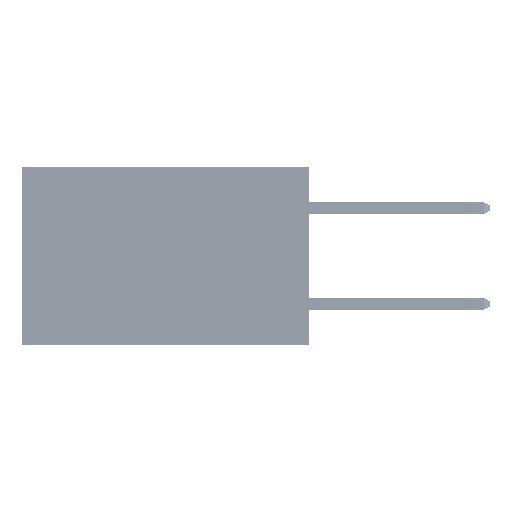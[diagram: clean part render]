
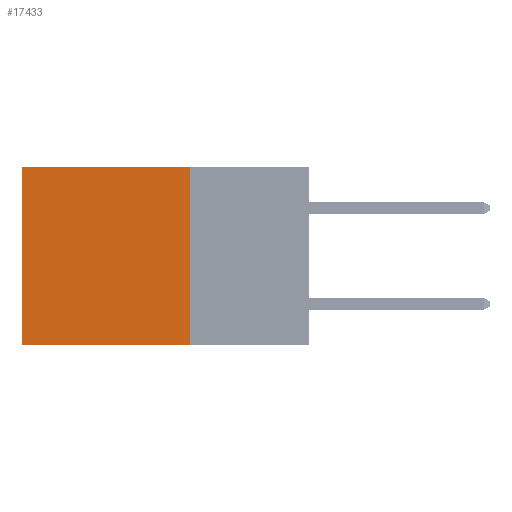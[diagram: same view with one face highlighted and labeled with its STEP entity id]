
A CAD part, left-side view. The second image highlights one B-rep face of the part: STEP entity #17433.
In plain terms, the highlighted planar face has unit normal (-1, 0, 0).
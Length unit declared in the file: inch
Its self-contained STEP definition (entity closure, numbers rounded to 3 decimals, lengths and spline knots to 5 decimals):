
#2884 = CARTESIAN_POINT ( 'NONE',  ( 0.2875, 0.25, -0.37 ) ) ;
#4389 = VERTEX_POINT ( 'NONE', #19653 ) ;
#5215 = DIRECTION ( 'NONE',  ( 0., 0., -1. ) ) ;
#7055 = CARTESIAN_POINT ( 'NONE',  ( 0.2875, 0.6, 0. ) ) ;
#9656 = DIRECTION ( 'NONE',  ( 0., 0., -1. ) ) ;
#12608 = DIRECTION ( 'NONE',  ( 1., 0., 0. ) ) ;
#12686 = VECTOR ( 'NONE', #9656, 39.37008 ) ;
#16348 = ORIENTED_EDGE ( 'NONE', *, *, #30618, .F. ) ;
#17033 = VECTOR ( 'NONE', #17422, 39.37008 ) ;
#17422 = DIRECTION ( 'NONE',  ( 0., 1., 0. ) ) ;
#17433 = ADVANCED_FACE ( 'NONE', ( #20223 ), #38358, .F. ) ;
#17789 = AXIS2_PLACEMENT_3D ( 'NONE', #30491, #12608, #5215 ) ;
#17885 = LINE ( 'NONE', #2884, #17033 ) ;
#19653 = CARTESIAN_POINT ( 'NONE',  ( 0.2875, 0.6, -0.37 ) ) ;
#20223 = FACE_OUTER_BOUND ( 'NONE', #42103, .T. ) ;
#23236 = CARTESIAN_POINT ( 'NONE',  ( 0.2875, 0.25, 0. ) ) ;
#23722 = ORIENTED_EDGE ( 'NONE', *, *, #43523, .T. ) ;
#24325 = CARTESIAN_POINT ( 'NONE',  ( 0.2875, 0.6, 0. ) ) ;
#25564 = VERTEX_POINT ( 'NONE', #24325 ) ;
#27021 = EDGE_CURVE ( 'NONE', #33050, #4389, #17885, .T. ) ;
#27784 = LINE ( 'NONE', #23236, #12686 ) ;
#28741 = CARTESIAN_POINT ( 'NONE',  ( 0.2875, 0.25, 0. ) ) ;
#30158 = VECTOR ( 'NONE', #32794, 39.37008 ) ;
#30491 = CARTESIAN_POINT ( 'NONE',  ( 0.2875, 0.25, 0. ) ) ;
#30618 = EDGE_CURVE ( 'NONE', #34963, #33050, #27784, .T. ) ;
#32387 = VECTOR ( 'NONE', #47013, 39.37008 ) ;
#32725 = LINE ( 'NONE', #36074, #32387 ) ;
#32794 = DIRECTION ( 'NONE',  ( 0., 0., -1. ) ) ;
#33050 = VERTEX_POINT ( 'NONE', #40724 ) ;
#34963 = VERTEX_POINT ( 'NONE', #28741 ) ;
#36074 = CARTESIAN_POINT ( 'NONE',  ( 0.2875, 0.25, 0. ) ) ;
#38358 = PLANE ( 'NONE',  #17789 ) ;
#39714 = LINE ( 'NONE', #7055, #30158 ) ;
#40519 = ORIENTED_EDGE ( 'NONE', *, *, #27021, .F. ) ;
#40724 = CARTESIAN_POINT ( 'NONE',  ( 0.2875, 0.25, -0.37 ) ) ;
#42103 = EDGE_LOOP ( 'NONE', ( #46255, #40519, #16348, #23722 ) ) ;
#43523 = EDGE_CURVE ( 'NONE', #34963, #25564, #32725, .T. ) ;
#44466 = EDGE_CURVE ( 'NONE', #25564, #4389, #39714, .T. ) ;
#46255 = ORIENTED_EDGE ( 'NONE', *, *, #44466, .T. ) ;
#47013 = DIRECTION ( 'NONE',  ( 0., 1., 0. ) ) ;
